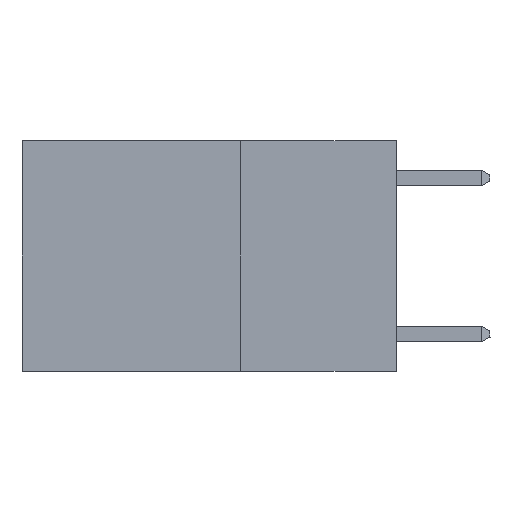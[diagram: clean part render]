
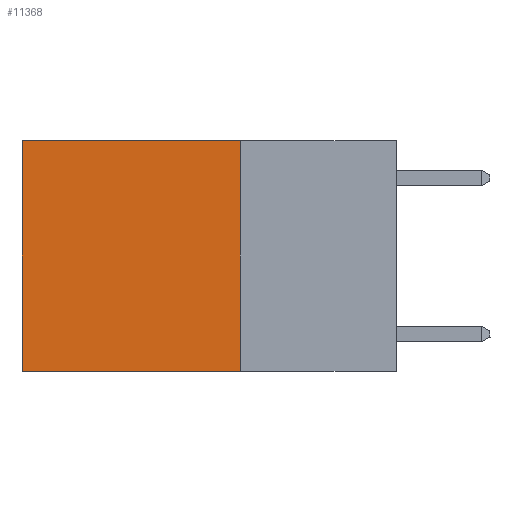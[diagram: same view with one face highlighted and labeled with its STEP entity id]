
A CAD part, left-side view. The second image highlights one B-rep face of the part: STEP entity #11368.
In plain terms, the highlighted planar face has unit normal (-1, 0, 0).
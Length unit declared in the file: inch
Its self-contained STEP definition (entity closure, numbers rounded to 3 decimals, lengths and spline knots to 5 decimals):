
#966 = ORIENTED_EDGE ( 'NONE', *, *, #20828, .T. ) ;
#1195 = ORIENTED_EDGE ( 'NONE', *, *, #21827, .F. ) ;
#1213 = ORIENTED_EDGE ( 'NONE', *, *, #2260, .F. ) ;
#1256 = ORIENTED_EDGE ( 'NONE', *, *, #5134, .T. ) ;
#2260 = EDGE_CURVE ( 'NONE', #11585, #12876, #3591, .T. ) ;
#2541 = CARTESIAN_POINT ( 'NONE',  ( 0.2625, 0.25, -0.37 ) ) ;
#3310 = VECTOR ( 'NONE', #10839, 39.37008 ) ;
#3567 = VECTOR ( 'NONE', #21138, 39.37008 ) ;
#3591 = LINE ( 'NONE', #21655, #3567 ) ;
#5134 = EDGE_CURVE ( 'NONE', #11585, #9144, #16950, .T. ) ;
#6176 = AXIS2_PLACEMENT_3D ( 'NONE', #13726, #6634, #18624 ) ;
#6634 = DIRECTION ( 'NONE',  ( 1., 0., 0. ) ) ;
#6896 = LINE ( 'NONE', #17366, #15678 ) ;
#7156 = CARTESIAN_POINT ( 'NONE',  ( 0.2625, 0.6, 0. ) ) ;
#9144 = VERTEX_POINT ( 'NONE', #15067 ) ;
#9277 = CARTESIAN_POINT ( 'NONE',  ( 0.2625, 0.6, -0.37 ) ) ;
#10622 = EDGE_LOOP ( 'NONE', ( #966, #1195, #1213, #1256 ) ) ;
#10839 = DIRECTION ( 'NONE',  ( 0., 0., -1. ) ) ;
#11368 = ADVANCED_FACE ( 'NONE', ( #15421 ), #12077, .F. ) ;
#11585 = VERTEX_POINT ( 'NONE', #12759 ) ;
#12077 = PLANE ( 'NONE',  #6176 ) ;
#12759 = CARTESIAN_POINT ( 'NONE',  ( 0.2625, 0.25, 0. ) ) ;
#12876 = VERTEX_POINT ( 'NONE', #2541 ) ;
#13726 = CARTESIAN_POINT ( 'NONE',  ( 0.2625, 0.25, 0. ) ) ;
#15067 = CARTESIAN_POINT ( 'NONE',  ( 0.2625, 0.6, 0. ) ) ;
#15421 = FACE_OUTER_BOUND ( 'NONE', #10622, .T. ) ;
#15475 = DIRECTION ( 'NONE',  ( 0., 1., 0. ) ) ;
#15557 = CARTESIAN_POINT ( 'NONE',  ( 0.2625, 0.25, 0. ) ) ;
#15678 = VECTOR ( 'NONE', #18952, 39.37008 ) ;
#16871 = VECTOR ( 'NONE', #15475, 39.37008 ) ;
#16950 = LINE ( 'NONE', #15557, #16871 ) ;
#17366 = CARTESIAN_POINT ( 'NONE',  ( 0.2625, 0.25, -0.37 ) ) ;
#17452 = LINE ( 'NONE', #7156, #3310 ) ;
#18624 = DIRECTION ( 'NONE',  ( 0., 0., -1. ) ) ;
#18952 = DIRECTION ( 'NONE',  ( 0., 1., 0. ) ) ;
#19957 = VERTEX_POINT ( 'NONE', #9277 ) ;
#20828 = EDGE_CURVE ( 'NONE', #9144, #19957, #17452, .T. ) ;
#21138 = DIRECTION ( 'NONE',  ( 0., 0., -1. ) ) ;
#21655 = CARTESIAN_POINT ( 'NONE',  ( 0.2625, 0.25, 0. ) ) ;
#21827 = EDGE_CURVE ( 'NONE', #12876, #19957, #6896, .T. ) ;
